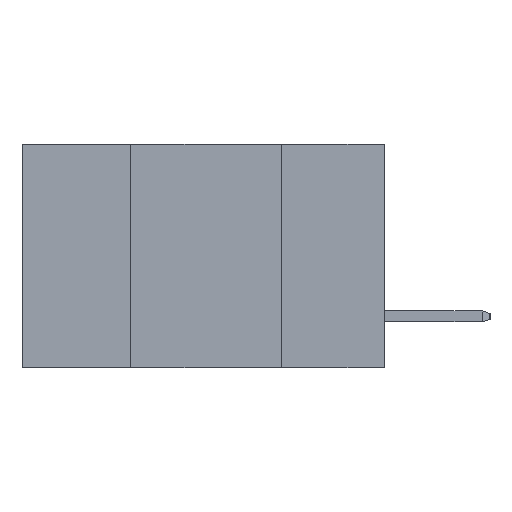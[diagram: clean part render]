
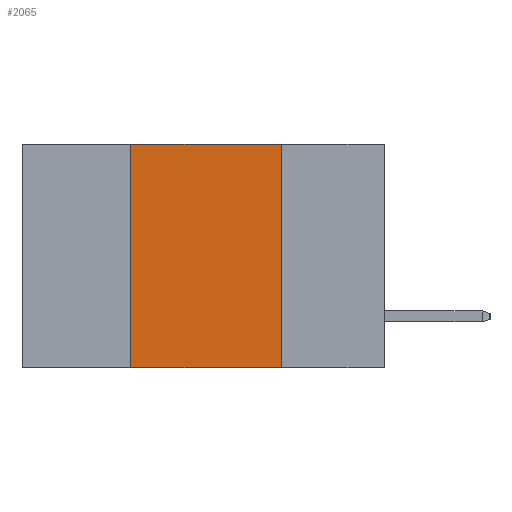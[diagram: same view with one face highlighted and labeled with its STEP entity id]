
A CAD part, left-side view. The second image highlights one B-rep face of the part: STEP entity #2065.
In plain terms, the highlighted planar face has unit normal (-1, 0, 0).
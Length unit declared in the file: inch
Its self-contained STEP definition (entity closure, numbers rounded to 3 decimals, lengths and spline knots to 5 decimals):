
#401 = EDGE_CURVE ( 'NONE', #9055, #1654, #6423, .T. ) ;
#674 = ORIENTED_EDGE ( 'NONE', *, *, #401, .F. ) ;
#688 = VECTOR ( 'NONE', #6181, 39.37008 ) ;
#1022 = LINE ( 'NONE', #6201, #688 ) ;
#1125 = EDGE_CURVE ( 'NONE', #3916, #9055, #12875, .T. ) ;
#1384 = CARTESIAN_POINT ( 'NONE',  ( 0., 0.17, 0. ) ) ;
#1654 = VERTEX_POINT ( 'NONE', #7884 ) ;
#1846 = EDGE_CURVE ( 'NONE', #12202, #3916, #1022, .T. ) ;
#2065 = ADVANCED_FACE ( 'NONE', ( #2997 ), #4198, .F. ) ;
#2162 = AXIS2_PLACEMENT_3D ( 'NONE', #4195, #4125, #4113 ) ;
#2326 = ORIENTED_EDGE ( 'NONE', *, *, #1846, .F. ) ;
#2551 = EDGE_CURVE ( 'NONE', #12202, #1654, #10112, .T. ) ;
#2997 = FACE_OUTER_BOUND ( 'NONE', #6297, .T. ) ;
#3210 = DIRECTION ( 'NONE',  ( 0., -1., 0. ) ) ;
#3813 = CARTESIAN_POINT ( 'NONE',  ( 0., 0.6, 0. ) ) ;
#3916 = VERTEX_POINT ( 'NONE', #10675 ) ;
#4113 = DIRECTION ( 'NONE',  ( 0., 0., -1. ) ) ;
#4125 = DIRECTION ( 'NONE',  ( 1., 0., 0. ) ) ;
#4195 = CARTESIAN_POINT ( 'NONE',  ( 0., 0.6, 0. ) ) ;
#4198 = PLANE ( 'NONE',  #2162 ) ;
#4781 = VECTOR ( 'NONE', #7159, 39.37008 ) ;
#4843 = CARTESIAN_POINT ( 'NONE',  ( 0., 0.42, -0.37 ) ) ;
#6181 = DIRECTION ( 'NONE',  ( 0., 0., 1. ) ) ;
#6201 = CARTESIAN_POINT ( 'NONE',  ( 0., 0.42, -0.37 ) ) ;
#6297 = EDGE_LOOP ( 'NONE', ( #674, #12383, #2326, #7769 ) ) ;
#6423 = LINE ( 'NONE', #11830, #8757 ) ;
#6806 = CARTESIAN_POINT ( 'NONE',  ( 0., 0.6, -0.37 ) ) ;
#7159 = DIRECTION ( 'NONE',  ( 0., -1., 0. ) ) ;
#7769 = ORIENTED_EDGE ( 'NONE', *, *, #2551, .T. ) ;
#7884 = CARTESIAN_POINT ( 'NONE',  ( 0., 0.17, -0.37 ) ) ;
#8757 = VECTOR ( 'NONE', #11817, 39.37008 ) ;
#9055 = VERTEX_POINT ( 'NONE', #1384 ) ;
#10112 = LINE ( 'NONE', #6806, #4781 ) ;
#10675 = CARTESIAN_POINT ( 'NONE',  ( 0., 0.42, 0. ) ) ;
#11817 = DIRECTION ( 'NONE',  ( 0., 0., -1. ) ) ;
#11830 = CARTESIAN_POINT ( 'NONE',  ( 0., 0.17, -0.37 ) ) ;
#12202 = VERTEX_POINT ( 'NONE', #4843 ) ;
#12271 = VECTOR ( 'NONE', #3210, 39.37008 ) ;
#12383 = ORIENTED_EDGE ( 'NONE', *, *, #1125, .F. ) ;
#12875 = LINE ( 'NONE', #3813, #12271 ) ;
